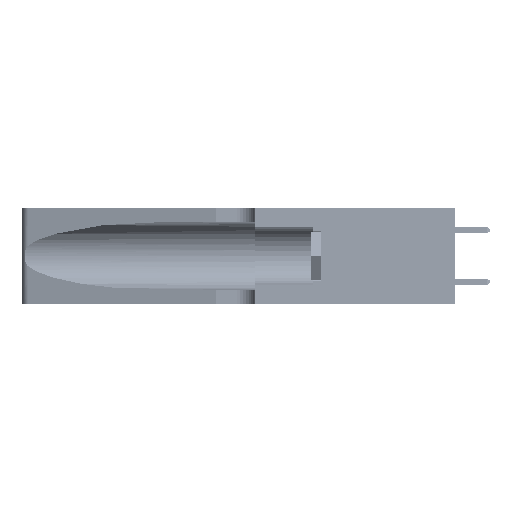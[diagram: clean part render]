
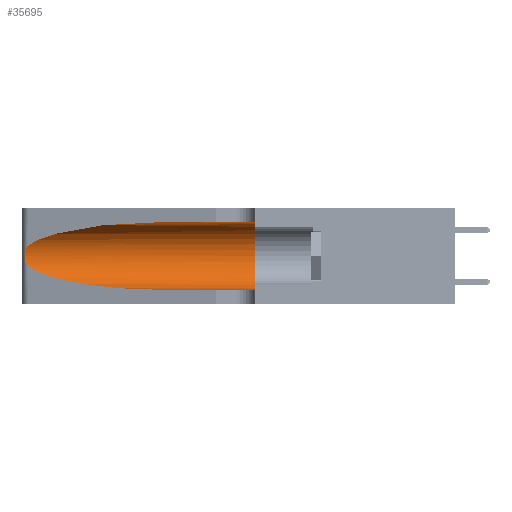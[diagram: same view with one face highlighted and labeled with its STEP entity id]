
A CAD part, left-side view. The second image highlights one B-rep face of the part: STEP entity #35695.
In plain terms, the highlighted cylindrical face has radius 3.308 mm (diameter 6.617 mm), a partial arc.
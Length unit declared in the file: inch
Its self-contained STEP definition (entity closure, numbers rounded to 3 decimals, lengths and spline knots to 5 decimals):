
#384 = EDGE_CURVE ( 'NONE', #21594, #29483, #9536, .T. ) ;
#1226 = EDGE_CURVE ( 'NONE', #29483, #28669, #22811, .T. ) ;
#2863 = CYLINDRICAL_SURFACE ( 'NONE', #18577, 0.13025 ) ;
#3518 = CARTESIAN_POINT ( 'NONE',  ( 0.26017, 1.23833, 0.17102 ) ) ;
#6990 = VECTOR ( 'NONE', #15313, 39.37008 ) ;
#7248 = CARTESIAN_POINT ( 'NONE',  ( 0.2373, 1.15595, 0.28018 ) ) ;
#7521 = ORIENTED_EDGE ( 'NONE', *, *, #46320, .T. ) ;
#7666 = CARTESIAN_POINT ( 'NONE',  ( 0.25789, 1.23486, 0.15765 ) ) ;
#7861 = ORIENTED_EDGE ( 'NONE', *, *, #39334, .T. ) ;
#9536 = LINE ( 'NONE', #35591, #6990 ) ;
#10456 = CARTESIAN_POINT ( 'NONE',  ( 0.1305, 1.61858, 0.185 ) ) ;
#11156 = CARTESIAN_POINT ( 'NONE',  ( 0.18966, 0.96281, 0.31525 ) ) ;
#11293 = CARTESIAN_POINT ( 'NONE',  ( 0.1305, 0.72297, 0.05475 ) ) ;
#11568 = CARTESIAN_POINT ( 'NONE',  ( 0.25487, 1.22718, 0.22369 ) ) ;
#11745 = CARTESIAN_POINT ( 'NONE',  ( 0.25555, 1.22993, 0.14849 ) ) ;
#12493 = DIRECTION ( 'NONE',  ( 0., 1., 0. ) ) ;
#13346 =( BOUNDED_CURVE ( )  B_SPLINE_CURVE ( 3, ( #36684, #20314, #48736, #40790 ),
 .UNSPECIFIED., .F., .F. ) 
 B_SPLINE_CURVE_WITH_KNOTS ( ( 4, 4 ),
 ( 3.44316, 4.71239 ),
 .UNSPECIFIED. ) 
 CURVE ( )  GEOMETRIC_REPRESENTATION_ITEM ( )  RATIONAL_B_SPLINE_CURVE ( ( 1., 0.87, 0.87, 1. ) ) 
 REPRESENTATION_ITEM ( '' )  );
#14575 = DIRECTION ( 'NONE',  ( 0., -1., 0. ) ) ;
#15075 = FACE_OUTER_BOUND ( 'NONE', #50403, .T. ) ;
#15182 = CARTESIAN_POINT ( 'NONE',  ( 0.25487, 1.22718, 0.14631 ) ) ;
#15313 = DIRECTION ( 'NONE',  ( 0., -1., 0. ) ) ;
#15963 = LINE ( 'NONE', #33440, #35054 ) ;
#18577 = AXIS2_PLACEMENT_3D ( 'NONE', #10456, #14575, #34864 ) ;
#19798 = CARTESIAN_POINT ( 'NONE',  ( 0.25787, 1.23484, 0.2124 ) ) ;
#19987 = AXIS2_PLACEMENT_3D ( 'NONE', #36893, #12493, #41003 ) ;
#20314 = CARTESIAN_POINT ( 'NONE',  ( 0.2373, 1.15595, 0.08982 ) ) ;
#20929 = ORIENTED_EDGE ( 'NONE', *, *, #384, .F. ) ;
#21594 = VERTEX_POINT ( 'NONE', #43158 ) ;
#22811 = CIRCLE ( 'NONE', #19987, 0.13025 ) ;
#23841 = CARTESIAN_POINT ( 'NONE',  ( 0.26018, 1.23835, 0.19895 ) ) ;
#27981 = CARTESIAN_POINT ( 'NONE',  ( 0.26075, 1.23896, 0.178 ) ) ;
#28084 = CARTESIAN_POINT ( 'NONE',  ( 0.1305, 0.35, 0.05475 ) ) ;
#28669 = VERTEX_POINT ( 'NONE', #28084 ) ;
#29077 = CARTESIAN_POINT ( 'NONE',  ( 0.1305, 0.35, 0.31525 ) ) ;
#29285 = ORIENTED_EDGE ( 'NONE', *, *, #40061, .T. ) ;
#29483 = VERTEX_POINT ( 'NONE', #29077 ) ;
#30561 = ORIENTED_EDGE ( 'NONE', *, *, #1226, .F. ) ;
#31204 = ORIENTED_EDGE ( 'NONE', *, *, #52021, .T. ) ;
#32098 = CARTESIAN_POINT ( 'NONE',  ( 0.25856, 1.23593, 0.16098 ) ) ;
#33440 = CARTESIAN_POINT ( 'NONE',  ( 0.1305, 1.61858, 0.05475 ) ) ;
#34864 = DIRECTION ( 'NONE',  ( 0., 0., -1. ) ) ;
#35054 = VECTOR ( 'NONE', #37511, 39.37008 ) ;
#35591 = CARTESIAN_POINT ( 'NONE',  ( 0.1305, 1.61858, 0.31525 ) ) ;
#35695 = ADVANCED_FACE ( 'NONE', ( #15075 ), #2863, .F. ) ;
#35751 = CARTESIAN_POINT ( 'NONE',  ( 0.25487, 1.22718, 0.22369 ) ) ;
#36165 = CARTESIAN_POINT ( 'NONE',  ( 0.25639, 1.23186, 0.15144 ) ) ;
#36684 = CARTESIAN_POINT ( 'NONE',  ( 0.25487, 1.22718, 0.14631 ) ) ;
#36893 = CARTESIAN_POINT ( 'NONE',  ( 0.1305, 0.35, 0.185 ) ) ;
#37511 = DIRECTION ( 'NONE',  ( 0., -1., 0. ) ) ;
#37829 = B_SPLINE_CURVE_WITH_KNOTS ( 'NONE', 3,
 ( #11568, #40112, #44143, #19798, #48223, #23841, #52293, #27981, #3518, #32098, #7666, #36165, #11745, #40285 ),
 .UNSPECIFIED., .F., .F.,
 ( 4, 2, 2, 2, 2, 2, 4 ),
 ( 0., 0.00027, 0.00053, 0.00107, 0.0016, 0.00187, 0.00214 ),
 .UNSPECIFIED. ) ;
#39137 = VERTEX_POINT ( 'NONE', #47694 ) ;
#39334 = EDGE_CURVE ( 'NONE', #43702, #41846, #13346, .T. ) ;
#40061 = EDGE_CURVE ( 'NONE', #41846, #28669, #15963, .T. ) ;
#40112 = CARTESIAN_POINT ( 'NONE',  ( 0.25555, 1.22994, 0.2215 ) ) ;
#40285 = CARTESIAN_POINT ( 'NONE',  ( 0.25487, 1.22718, 0.14631 ) ) ;
#40790 = CARTESIAN_POINT ( 'NONE',  ( 0.1305, 0.72297, 0.05475 ) ) ;
#41003 = DIRECTION ( 'NONE',  ( 0., 0., 1. ) ) ;
#41846 = VERTEX_POINT ( 'NONE', #11293 ) ;
#43158 = CARTESIAN_POINT ( 'NONE',  ( 0.1305, 0.72297, 0.31525 ) ) ;
#43702 = VERTEX_POINT ( 'NONE', #15182 ) ;
#44143 = CARTESIAN_POINT ( 'NONE',  ( 0.25639, 1.23184, 0.21858 ) ) ;
#46320 = EDGE_CURVE ( 'NONE', #21594, #39137, #47261, .T. ) ;
#47261 =( BOUNDED_CURVE ( )  B_SPLINE_CURVE ( 3, ( #51882, #11156, #7248, #35751 ),
 .UNSPECIFIED., .F., .F. ) 
 B_SPLINE_CURVE_WITH_KNOTS ( ( 4, 4 ),
 ( 1.5708, 2.84003 ),
 .UNSPECIFIED. ) 
 CURVE ( )  GEOMETRIC_REPRESENTATION_ITEM ( )  RATIONAL_B_SPLINE_CURVE ( ( 1., 0.87, 0.87, 1. ) ) 
 REPRESENTATION_ITEM ( '' )  );
#47694 = CARTESIAN_POINT ( 'NONE',  ( 0.25487, 1.22718, 0.22369 ) ) ;
#48223 = CARTESIAN_POINT ( 'NONE',  ( 0.25854, 1.2359, 0.20912 ) ) ;
#48736 = CARTESIAN_POINT ( 'NONE',  ( 0.18966, 0.96281, 0.05475 ) ) ;
#50403 = EDGE_LOOP ( 'NONE', ( #7521, #31204, #7861, #29285, #30561, #20929 ) ) ;
#51882 = CARTESIAN_POINT ( 'NONE',  ( 0.1305, 0.72297, 0.31525 ) ) ;
#52021 = EDGE_CURVE ( 'NONE', #39137, #43702, #37829, .T. ) ;
#52293 = CARTESIAN_POINT ( 'NONE',  ( 0.26075, 1.23896, 0.19203 ) ) ;
